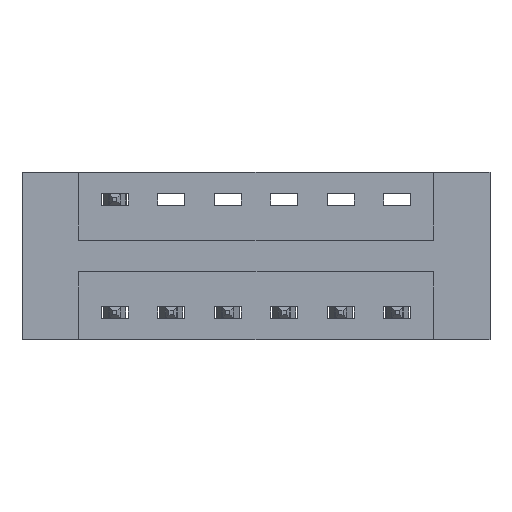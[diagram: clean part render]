
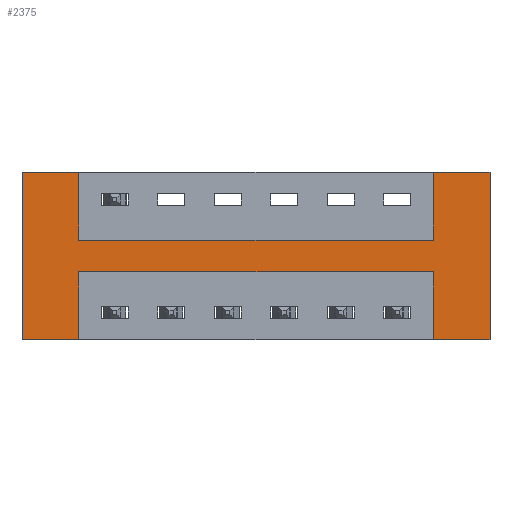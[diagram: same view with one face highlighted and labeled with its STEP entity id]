
A CAD part, front view. The second image highlights one B-rep face of the part: STEP entity #2375.
In plain terms, the highlighted planar face has unit normal (0, -1, 0).
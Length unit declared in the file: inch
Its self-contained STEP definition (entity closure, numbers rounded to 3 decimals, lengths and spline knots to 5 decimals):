
#4 = DIRECTION ( 'NONE',  ( 0., 0., -1. ) ) ;
#120 = LINE ( 'NONE', #1686, #5230 ) ;
#229 = LINE ( 'NONE', #1409, #1870 ) ;
#269 = CARTESIAN_POINT ( 'NONE',  ( 1.2975, 0., 0. ) ) ;
#356 = VECTOR ( 'NONE', #6618, 39.37008 ) ;
#357 = CARTESIAN_POINT ( 'NONE',  ( 0., 0., -0.37 ) ) ;
#439 = VERTEX_POINT ( 'NONE', #3805 ) ;
#442 = VECTOR ( 'NONE', #3709, 39.37008 ) ;
#592 = CARTESIAN_POINT ( 'NONE',  ( 0.2625, 0., -0.37 ) ) ;
#640 = LINE ( 'NONE', #2093, #3861 ) ;
#660 = VERTEX_POINT ( 'NONE', #5224 ) ;
#663 = CARTESIAN_POINT ( 'NONE',  ( 0., 0., 0. ) ) ;
#685 = VERTEX_POINT ( 'NONE', #2757 ) ;
#701 = VERTEX_POINT ( 'NONE', #5903 ) ;
#739 = ORIENTED_EDGE ( 'NONE', *, *, #7085, .T. ) ;
#768 = CARTESIAN_POINT ( 'NONE',  ( 0.3875, 0., 0. ) ) ;
#798 = VERTEX_POINT ( 'NONE', #3549 ) ;
#823 = ORIENTED_EDGE ( 'NONE', *, *, #5361, .F. ) ;
#868 = ORIENTED_EDGE ( 'NONE', *, *, #7616, .F. ) ;
#1053 = ORIENTED_EDGE ( 'NONE', *, *, #1187, .F. ) ;
#1078 = ORIENTED_EDGE ( 'NONE', *, *, #7899, .F. ) ;
#1187 = EDGE_CURVE ( 'NONE', #439, #3344, #1665, .T. ) ;
#1367 = CARTESIAN_POINT ( 'NONE',  ( 0., 0., -0.37 ) ) ;
#1409 = CARTESIAN_POINT ( 'NONE',  ( 1.1725, 0., 0. ) ) ;
#1556 = ORIENTED_EDGE ( 'NONE', *, *, #2357, .F. ) ;
#1665 = LINE ( 'NONE', #5941, #5153 ) ;
#1686 = CARTESIAN_POINT ( 'NONE',  ( 0.3875, 0., 0. ) ) ;
#1711 = ORIENTED_EDGE ( 'NONE', *, *, #7584, .T. ) ;
#1718 = DIRECTION ( 'NONE',  ( 0., 0., -1. ) ) ;
#1764 = PLANE ( 'NONE',  #6223 ) ;
#1766 = ORIENTED_EDGE ( 'NONE', *, *, #3311, .F. ) ;
#1837 = VERTEX_POINT ( 'NONE', #7509 ) ;
#1870 = VECTOR ( 'NONE', #2131, 39.37008 ) ;
#1880 = ORIENTED_EDGE ( 'NONE', *, *, #5630, .F. ) ;
#1925 = ORIENTED_EDGE ( 'NONE', *, *, #3247, .F. ) ;
#2067 = CARTESIAN_POINT ( 'NONE',  ( 1.1725, 0., 0. ) ) ;
#2093 = CARTESIAN_POINT ( 'NONE',  ( 0.2625, 0., 0. ) ) ;
#2099 = LINE ( 'NONE', #269, #442 ) ;
#2129 = DIRECTION ( 'NONE',  ( 1., 0., 0. ) ) ;
#2131 = DIRECTION ( 'NONE',  ( 0., 0., 1. ) ) ;
#2156 = ORIENTED_EDGE ( 'NONE', *, *, #2454, .F. ) ;
#2357 = EDGE_CURVE ( 'NONE', #7471, #3469, #8217, .T. ) ;
#2375 = ADVANCED_FACE ( 'NONE', ( #6353 ), #1764, .T. ) ;
#2454 = EDGE_CURVE ( 'NONE', #685, #7776, #3763, .T. ) ;
#2483 = DIRECTION ( 'NONE',  ( 0., -1., 0. ) ) ;
#2757 = CARTESIAN_POINT ( 'NONE',  ( 1.1725, 0., -0.37 ) ) ;
#2771 = ORIENTED_EDGE ( 'NONE', *, *, #6418, .F. ) ;
#2876 = VERTEX_POINT ( 'NONE', #2067 ) ;
#2916 = CARTESIAN_POINT ( 'NONE',  ( 0., 0., 0. ) ) ;
#3236 = VERTEX_POINT ( 'NONE', #592 ) ;
#3247 = EDGE_CURVE ( 'NONE', #7776, #1837, #3640, .T. ) ;
#3306 = DIRECTION ( 'NONE',  ( 0., 0., 1. ) ) ;
#3311 = EDGE_CURVE ( 'NONE', #660, #3236, #6883, .T. ) ;
#3344 = VERTEX_POINT ( 'NONE', #7168 ) ;
#3469 = VERTEX_POINT ( 'NONE', #768 ) ;
#3549 = CARTESIAN_POINT ( 'NONE',  ( 1.2975, 0., -0.37 ) ) ;
#3609 = VECTOR ( 'NONE', #5909, 39.37008 ) ;
#3640 = LINE ( 'NONE', #4622, #6708 ) ;
#3709 = DIRECTION ( 'NONE',  ( 0., 0., 1. ) ) ;
#3763 = LINE ( 'NONE', #6989, #5416 ) ;
#3805 = CARTESIAN_POINT ( 'NONE',  ( 0.3875, 0., -0.15 ) ) ;
#3858 = CARTESIAN_POINT ( 'NONE',  ( 0., 0., -0.37 ) ) ;
#3861 = VECTOR ( 'NONE', #4, 39.37008 ) ;
#4238 = LINE ( 'NONE', #6807, #5518 ) ;
#4622 = CARTESIAN_POINT ( 'NONE',  ( 0.3875, 0., -0.22 ) ) ;
#5049 = EDGE_LOOP ( 'NONE', ( #739, #823, #868, #1053, #1078, #1556, #1711, #1766, #1880, #1925, #2156, #2771 ) ) ;
#5117 = DIRECTION ( 'NONE',  ( -1., 0., 0. ) ) ;
#5153 = VECTOR ( 'NONE', #2129, 39.37008 ) ;
#5224 = CARTESIAN_POINT ( 'NONE',  ( 0.3875, 0., -0.37 ) ) ;
#5230 = VECTOR ( 'NONE', #7381, 39.37008 ) ;
#5361 = EDGE_CURVE ( 'NONE', #2876, #701, #7250, .T. ) ;
#5416 = VECTOR ( 'NONE', #3306, 39.37008 ) ;
#5518 = VECTOR ( 'NONE', #1718, 39.37008 ) ;
#5630 = EDGE_CURVE ( 'NONE', #1837, #660, #4238, .T. ) ;
#5845 = CARTESIAN_POINT ( 'NONE',  ( 0.2625, 0., 0. ) ) ;
#5903 = CARTESIAN_POINT ( 'NONE',  ( 1.2975, 0., 0. ) ) ;
#5907 = VECTOR ( 'NONE', #5117, 39.37008 ) ;
#5909 = DIRECTION ( 'NONE',  ( -1., 0., 0. ) ) ;
#5941 = CARTESIAN_POINT ( 'NONE',  ( 0.3875, 0., -0.15 ) ) ;
#6041 = CARTESIAN_POINT ( 'NONE',  ( 1.1725, 0., -0.22 ) ) ;
#6223 = AXIS2_PLACEMENT_3D ( 'NONE', #357, #2483, #6849 ) ;
#6353 = FACE_OUTER_BOUND ( 'NONE', #5049, .T. ) ;
#6418 = EDGE_CURVE ( 'NONE', #798, #685, #7534, .T. ) ;
#6543 = VECTOR ( 'NONE', #7420, 39.37008 ) ;
#6618 = DIRECTION ( 'NONE',  ( 1., 0., 0. ) ) ;
#6708 = VECTOR ( 'NONE', #7082, 39.37008 ) ;
#6807 = CARTESIAN_POINT ( 'NONE',  ( 0.3875, 0., -0.37 ) ) ;
#6849 = DIRECTION ( 'NONE',  ( 0., 0., -1. ) ) ;
#6883 = LINE ( 'NONE', #1367, #3609 ) ;
#6989 = CARTESIAN_POINT ( 'NONE',  ( 1.1725, 0., -0.37 ) ) ;
#7082 = DIRECTION ( 'NONE',  ( -1., 0., 0. ) ) ;
#7085 = EDGE_CURVE ( 'NONE', #798, #701, #2099, .T. ) ;
#7168 = CARTESIAN_POINT ( 'NONE',  ( 1.1725, 0., -0.15 ) ) ;
#7250 = LINE ( 'NONE', #2916, #356 ) ;
#7381 = DIRECTION ( 'NONE',  ( 0., 0., -1. ) ) ;
#7420 = DIRECTION ( 'NONE',  ( 1., 0., 0. ) ) ;
#7471 = VERTEX_POINT ( 'NONE', #5845 ) ;
#7509 = CARTESIAN_POINT ( 'NONE',  ( 0.3875, 0., -0.22 ) ) ;
#7534 = LINE ( 'NONE', #3858, #5907 ) ;
#7584 = EDGE_CURVE ( 'NONE', #7471, #3236, #640, .T. ) ;
#7616 = EDGE_CURVE ( 'NONE', #3344, #2876, #229, .T. ) ;
#7776 = VERTEX_POINT ( 'NONE', #6041 ) ;
#7899 = EDGE_CURVE ( 'NONE', #3469, #439, #120, .T. ) ;
#8217 = LINE ( 'NONE', #663, #6543 ) ;
